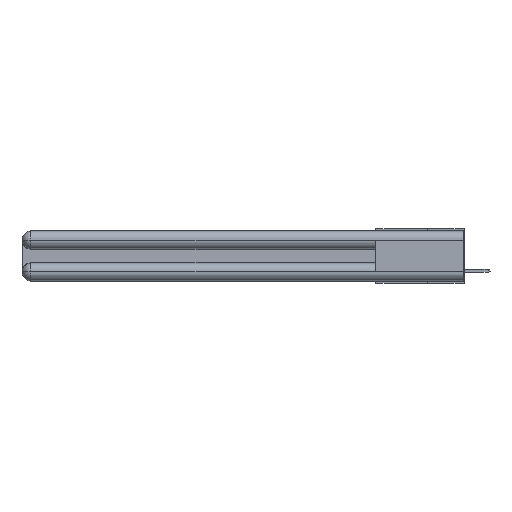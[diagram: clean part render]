
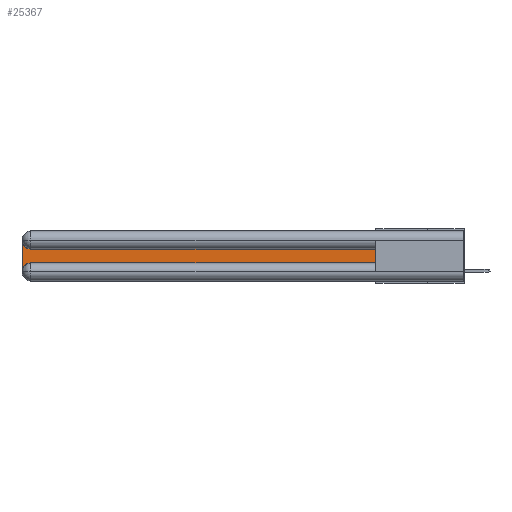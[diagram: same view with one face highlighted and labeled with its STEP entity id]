
A CAD part, left-side view. The second image highlights one B-rep face of the part: STEP entity #25367.
In plain terms, the highlighted planar face has unit normal (-1, 0, 0).
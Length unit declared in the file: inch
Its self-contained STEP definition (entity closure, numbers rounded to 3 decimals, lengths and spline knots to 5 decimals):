
#631 = DIRECTION ( 'NONE',  ( 1., 0., 0. ) ) ;
#742 = VERTEX_POINT ( 'NONE', #2623 ) ;
#1048 = DIRECTION ( 'NONE',  ( 0., -1., 0. ) ) ;
#1158 = VECTOR ( 'NONE', #1048, 39.37008 ) ;
#1283 = CARTESIAN_POINT ( 'NONE',  ( 0.075, 0.6, -0.2175 ) ) ;
#1466 = CARTESIAN_POINT ( 'NONE',  ( 0.075, 0.6, -0.2175 ) ) ;
#1702 = DIRECTION ( 'NONE',  ( 0., 0., -1. ) ) ;
#2069 = AXIS2_PLACEMENT_3D ( 'NONE', #8311, #631, #16401 ) ;
#2257 = PLANE ( 'NONE',  #16761 ) ;
#2479 = DIRECTION ( 'NONE',  ( 0., 0., -1. ) ) ;
#2623 = CARTESIAN_POINT ( 'NONE',  ( 0.075, 3., -0.2775 ) ) ;
#3016 = ORIENTED_EDGE ( 'NONE', *, *, #6777, .T. ) ;
#3852 = ORIENTED_EDGE ( 'NONE', *, *, #23666, .T. ) ;
#4628 = CARTESIAN_POINT ( 'NONE',  ( 0.075, 3., -0.2175 ) ) ;
#6326 = DIRECTION ( 'NONE',  ( 0., 1., 0. ) ) ;
#6558 = CIRCLE ( 'NONE', #2069, 0.06 ) ;
#6777 = EDGE_CURVE ( 'NONE', #17453, #742, #16967, .T. ) ;
#7235 = EDGE_LOOP ( 'NONE', ( #7475, #3852, #3016, #10085, #9565, #28491 ) ) ;
#7475 = ORIENTED_EDGE ( 'NONE', *, *, #27874, .T. ) ;
#8156 = CARTESIAN_POINT ( 'NONE',  ( 0.075, 3., -0.0625 ) ) ;
#8311 = CARTESIAN_POINT ( 'NONE',  ( 0.075, 2.94, -0.0625 ) ) ;
#9311 = VERTEX_POINT ( 'NONE', #13003 ) ;
#9565 = ORIENTED_EDGE ( 'NONE', *, *, #10153, .T. ) ;
#9680 = DIRECTION ( 'NONE',  ( 0., 0., 1. ) ) ;
#10085 = ORIENTED_EDGE ( 'NONE', *, *, #31908, .T. ) ;
#10153 = EDGE_CURVE ( 'NONE', #9311, #27543, #31006, .T. ) ;
#11416 = AXIS2_PLACEMENT_3D ( 'NONE', #32916, #14693, #1702 ) ;
#12747 = DIRECTION ( 'NONE',  ( 1., 0., 0. ) ) ;
#13003 = CARTESIAN_POINT ( 'NONE',  ( 0.075, 2.94, -0.2175 ) ) ;
#13699 = CARTESIAN_POINT ( 'NONE',  ( 0.075, 0.6, -0.1225 ) ) ;
#14693 = DIRECTION ( 'NONE',  ( 1., 0., 0. ) ) ;
#14757 = CIRCLE ( 'NONE', #11416, 0.06 ) ;
#16401 = DIRECTION ( 'NONE',  ( 0., 0., -1. ) ) ;
#16463 = CARTESIAN_POINT ( 'NONE',  ( 0.075, 0.6, -0.1225 ) ) ;
#16761 = AXIS2_PLACEMENT_3D ( 'NONE', #31298, #12747, #2479 ) ;
#16967 = LINE ( 'NONE', #4628, #30071 ) ;
#17203 = LINE ( 'NONE', #1466, #29075 ) ;
#17453 = VERTEX_POINT ( 'NONE', #8156 ) ;
#17762 = EDGE_CURVE ( 'NONE', #27543, #21451, #17203, .T. ) ;
#21451 = VERTEX_POINT ( 'NONE', #13699 ) ;
#23666 = EDGE_CURVE ( 'NONE', #24284, #17453, #6558, .T. ) ;
#24284 = VERTEX_POINT ( 'NONE', #30068 ) ;
#25367 = ADVANCED_FACE ( 'NONE', ( #29322 ), #2257, .F. ) ;
#25498 = LINE ( 'NONE', #16463, #30832 ) ;
#27543 = VERTEX_POINT ( 'NONE', #33549 ) ;
#27874 = EDGE_CURVE ( 'NONE', #21451, #24284, #25498, .T. ) ;
#28491 = ORIENTED_EDGE ( 'NONE', *, *, #17762, .T. ) ;
#29075 = VECTOR ( 'NONE', #9680, 39.37008 ) ;
#29146 = DIRECTION ( 'NONE',  ( 0., 0., -1. ) ) ;
#29322 = FACE_OUTER_BOUND ( 'NONE', #7235, .T. ) ;
#30068 = CARTESIAN_POINT ( 'NONE',  ( 0.075, 2.94, -0.1225 ) ) ;
#30071 = VECTOR ( 'NONE', #29146, 39.37008 ) ;
#30832 = VECTOR ( 'NONE', #6326, 39.37008 ) ;
#31006 = LINE ( 'NONE', #1283, #1158 ) ;
#31298 = CARTESIAN_POINT ( 'NONE',  ( 0.075, 3., -0.1225 ) ) ;
#31908 = EDGE_CURVE ( 'NONE', #742, #9311, #14757, .T. ) ;
#32916 = CARTESIAN_POINT ( 'NONE',  ( 0.075, 2.94, -0.2775 ) ) ;
#33549 = CARTESIAN_POINT ( 'NONE',  ( 0.075, 0.6, -0.2175 ) ) ;
